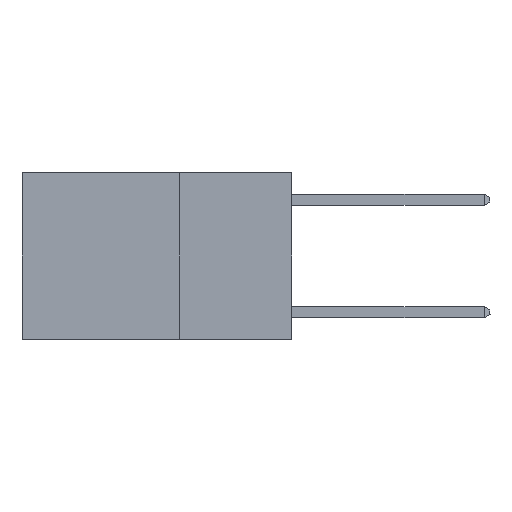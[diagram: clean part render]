
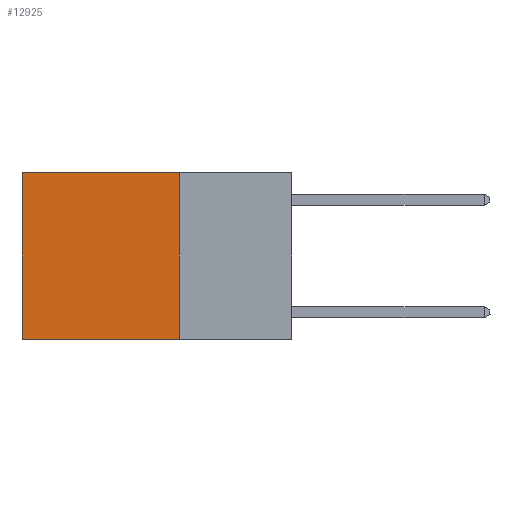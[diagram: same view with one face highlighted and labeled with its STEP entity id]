
A CAD part, left-side view. The second image highlights one B-rep face of the part: STEP entity #12925.
In plain terms, the highlighted planar face has unit normal (-1, 0, 0).
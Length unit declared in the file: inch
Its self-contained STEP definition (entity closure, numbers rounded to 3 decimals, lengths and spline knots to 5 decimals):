
#66 = CARTESIAN_POINT ( 'NONE',  ( 0.2625, 0.6, 0. ) ) ;
#494 = CARTESIAN_POINT ( 'NONE',  ( 0.2625, 0.25, -0.37 ) ) ;
#1342 = DIRECTION ( 'NONE',  ( 1., 0., 0. ) ) ;
#1626 = ORIENTED_EDGE ( 'NONE', *, *, #16379, .T. ) ;
#2501 = VERTEX_POINT ( 'NONE', #494 ) ;
#2621 = CARTESIAN_POINT ( 'NONE',  ( 0.2625, 0.25, 0. ) ) ;
#3286 = EDGE_CURVE ( 'NONE', #2501, #16947, #4496, .T. ) ;
#3859 = EDGE_CURVE ( 'NONE', #8332, #2501, #17786, .T. ) ;
#3992 = EDGE_CURVE ( 'NONE', #11547, #16947, #12301, .T. ) ;
#3994 = VECTOR ( 'NONE', #16421, 39.37008 ) ;
#3997 = CARTESIAN_POINT ( 'NONE',  ( 0.2625, 0.6, 0. ) ) ;
#4086 = ORIENTED_EDGE ( 'NONE', *, *, #3992, .T. ) ;
#4496 = LINE ( 'NONE', #5874, #13003 ) ;
#5040 = VECTOR ( 'NONE', #7486, 39.37008 ) ;
#5619 = DIRECTION ( 'NONE',  ( 0., 0., -1. ) ) ;
#5874 = CARTESIAN_POINT ( 'NONE',  ( 0.2625, 0.25, -0.37 ) ) ;
#5940 = LINE ( 'NONE', #11329, #5040 ) ;
#6107 = ORIENTED_EDGE ( 'NONE', *, *, #3859, .F. ) ;
#6828 = ORIENTED_EDGE ( 'NONE', *, *, #3286, .F. ) ;
#7486 = DIRECTION ( 'NONE',  ( 0., 1., 0. ) ) ;
#7922 = CARTESIAN_POINT ( 'NONE',  ( 0.2625, 0.6, -0.37 ) ) ;
#8332 = VERTEX_POINT ( 'NONE', #18002 ) ;
#8757 = EDGE_LOOP ( 'NONE', ( #4086, #6828, #6107, #1626 ) ) ;
#10389 = VECTOR ( 'NONE', #17872, 39.37008 ) ;
#11329 = CARTESIAN_POINT ( 'NONE',  ( 0.2625, 0.25, 0. ) ) ;
#11437 = DIRECTION ( 'NONE',  ( 0., 1., 0. ) ) ;
#11547 = VERTEX_POINT ( 'NONE', #66 ) ;
#12301 = LINE ( 'NONE', #3997, #10389 ) ;
#12925 = ADVANCED_FACE ( 'NONE', ( #13928 ), #15389, .F. ) ;
#13003 = VECTOR ( 'NONE', #11437, 39.37008 ) ;
#13423 = CARTESIAN_POINT ( 'NONE',  ( 0.2625, 0.25, 0. ) ) ;
#13928 = FACE_OUTER_BOUND ( 'NONE', #8757, .T. ) ;
#15389 = PLANE ( 'NONE',  #15759 ) ;
#15759 = AXIS2_PLACEMENT_3D ( 'NONE', #2621, #1342, #5619 ) ;
#16379 = EDGE_CURVE ( 'NONE', #8332, #11547, #5940, .T. ) ;
#16421 = DIRECTION ( 'NONE',  ( 0., 0., -1. ) ) ;
#16947 = VERTEX_POINT ( 'NONE', #7922 ) ;
#17786 = LINE ( 'NONE', #13423, #3994 ) ;
#17872 = DIRECTION ( 'NONE',  ( 0., 0., -1. ) ) ;
#18002 = CARTESIAN_POINT ( 'NONE',  ( 0.2625, 0.25, 0. ) ) ;
